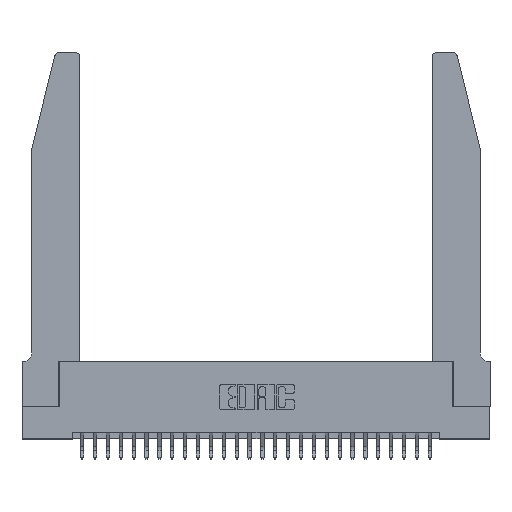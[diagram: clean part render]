
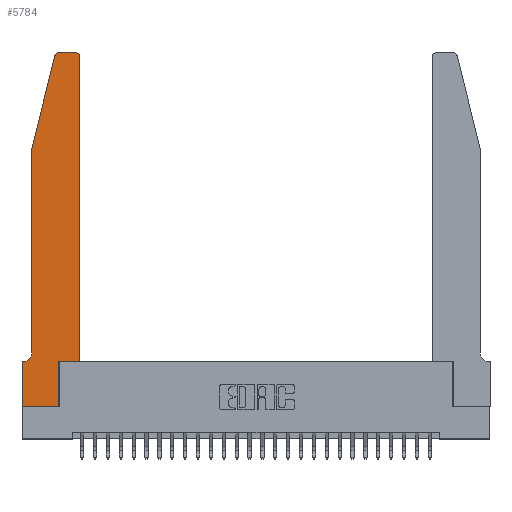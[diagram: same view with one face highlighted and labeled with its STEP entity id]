
A CAD part, top view. The second image highlights one B-rep face of the part: STEP entity #5784.
In plain terms, the highlighted planar face has unit normal (0, 0, 1).
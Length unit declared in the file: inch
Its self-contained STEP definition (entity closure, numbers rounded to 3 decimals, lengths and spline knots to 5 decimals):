
#33 = DIRECTION ( 'NONE',  ( 0., 1., 0. ) ) ;
#262 = VECTOR ( 'NONE', #13490, 39.37008 ) ;
#275 = ORIENTED_EDGE ( 'NONE', *, *, #11122, .T. ) ;
#571 = VERTEX_POINT ( 'NONE', #5229 ) ;
#741 = VERTEX_POINT ( 'NONE', #20770 ) ;
#930 = LINE ( 'NONE', #17009, #28403 ) ;
#1021 = ORIENTED_EDGE ( 'NONE', *, *, #4474, .T. ) ;
#1080 = FACE_OUTER_BOUND ( 'NONE', #5150, .T. ) ;
#1816 = CARTESIAN_POINT ( 'NONE',  ( 0.2865, 0.35, 0.37 ) ) ;
#1835 = CIRCLE ( 'NONE', #12754, 0.03 ) ;
#1891 = LINE ( 'NONE', #13065, #13332 ) ;
#2243 = LINE ( 'NONE', #26798, #19398 ) ;
#4474 = EDGE_CURVE ( 'NONE', #21054, #741, #24254, .T. ) ;
#4695 = CARTESIAN_POINT ( 'NONE',  ( 0., 0.35, 0.37 ) ) ;
#5145 = ORIENTED_EDGE ( 'NONE', *, *, #24065, .T. ) ;
#5150 = EDGE_LOOP ( 'NONE', ( #5145, #16934, #22730, #275, #1021, #7296, #18976, #20340, #15926, #21708, #11509, #28837 ) ) ;
#5229 = CARTESIAN_POINT ( 'NONE',  ( 0.4505, 0.35, 0.37 ) ) ;
#5756 = VECTOR ( 'NONE', #20949, 39.37008 ) ;
#5784 = ADVANCED_FACE ( 'NONE', ( #1080 ), #17998, .T. ) ;
#6334 = CARTESIAN_POINT ( 'NONE',  ( 0.4205, 2.72, 0.37 ) ) ;
#6457 = EDGE_CURVE ( 'NONE', #17022, #22166, #13598, .T. ) ;
#7056 = CARTESIAN_POINT ( 'NONE',  ( 0.0755, 2., 0.37 ) ) ;
#7296 = ORIENTED_EDGE ( 'NONE', *, *, #10731, .T. ) ;
#7402 = CIRCLE ( 'NONE', #26269, 0.03 ) ;
#7629 = VECTOR ( 'NONE', #26615, 39.37008 ) ;
#7757 = CARTESIAN_POINT ( 'NONE',  ( 0.4505, 0.35, 0.37 ) ) ;
#8223 = CARTESIAN_POINT ( 'NONE',  ( 0., 0.35, 0.37 ) ) ;
#8578 = DIRECTION ( 'NONE',  ( 1., 0., 0. ) ) ;
#9175 = CARTESIAN_POINT ( 'NONE',  ( 0.4505, 2.72, 0.37 ) ) ;
#9250 = DIRECTION ( 'NONE',  ( 0., 0., 1. ) ) ;
#9281 = DIRECTION ( 'NONE',  ( 0., -1., 0. ) ) ;
#9647 = EDGE_CURVE ( 'NONE', #571, #27584, #28255, .T. ) ;
#10397 = CARTESIAN_POINT ( 'NONE',  ( 0.0755, 0.42, 0.37 ) ) ;
#10710 = VERTEX_POINT ( 'NONE', #22911 ) ;
#10731 = EDGE_CURVE ( 'NONE', #741, #17732, #26187, .T. ) ;
#10800 = CARTESIAN_POINT ( 'NONE',  ( 0.0755, 2., 0.37 ) ) ;
#11122 = EDGE_CURVE ( 'NONE', #22166, #21054, #15287, .T. ) ;
#11227 = CARTESIAN_POINT ( 'NONE',  ( 0., 0., 0.37 ) ) ;
#11301 = CARTESIAN_POINT ( 'NONE',  ( 0.0755, 2., 0.37 ) ) ;
#11402 = CARTESIAN_POINT ( 'NONE',  ( 0.0055, 0.42, 0.37 ) ) ;
#11509 = ORIENTED_EDGE ( 'NONE', *, *, #9647, .T. ) ;
#11668 = EDGE_CURVE ( 'NONE', #17732, #14678, #12518, .T. ) ;
#12518 = LINE ( 'NONE', #11227, #262 ) ;
#12657 = DIRECTION ( 'NONE',  ( 1., 0., 0. ) ) ;
#12754 = AXIS2_PLACEMENT_3D ( 'NONE', #6334, #21676, #8578 ) ;
#13065 = CARTESIAN_POINT ( 'NONE',  ( 0.2605, 2.75, 0.37 ) ) ;
#13214 = CARTESIAN_POINT ( 'NONE',  ( 0.284, 2.72, 0.37 ) ) ;
#13332 = VECTOR ( 'NONE', #23901, 39.37008 ) ;
#13468 = EDGE_CURVE ( 'NONE', #22896, #571, #17512, .T. ) ;
#13490 = DIRECTION ( 'NONE',  ( 0., -1., 0. ) ) ;
#13598 = LINE ( 'NONE', #11301, #7629 ) ;
#13644 = DIRECTION ( 'NONE',  ( -1., 0., 0. ) ) ;
#13723 = AXIS2_PLACEMENT_3D ( 'NONE', #4695, #9250, #24584 ) ;
#14387 = CARTESIAN_POINT ( 'NONE',  ( 0., 0., 0.37 ) ) ;
#14611 = VECTOR ( 'NONE', #9281, 39.37008 ) ;
#14678 = VERTEX_POINT ( 'NONE', #14387 ) ;
#15287 = LINE ( 'NONE', #7056, #14611 ) ;
#15385 = DIRECTION ( 'NONE',  ( 1., 0., 0. ) ) ;
#15926 = ORIENTED_EDGE ( 'NONE', *, *, #24286, .T. ) ;
#16827 = CARTESIAN_POINT ( 'NONE',  ( 0.25487, 2.72718, 0.37 ) ) ;
#16934 = ORIENTED_EDGE ( 'NONE', *, *, #17890, .T. ) ;
#17009 = CARTESIAN_POINT ( 'NONE',  ( 0., 0., 0.37 ) ) ;
#17022 = VERTEX_POINT ( 'NONE', #16827 ) ;
#17398 = VECTOR ( 'NONE', #23135, 39.37008 ) ;
#17512 = LINE ( 'NONE', #18769, #5756 ) ;
#17590 = AXIS2_PLACEMENT_3D ( 'NONE', #11402, #26620, #13644 ) ;
#17732 = VERTEX_POINT ( 'NONE', #8223 ) ;
#17890 = EDGE_CURVE ( 'NONE', #10710, #17022, #7402, .T. ) ;
#17998 = PLANE ( 'NONE',  #13723 ) ;
#18326 = VERTEX_POINT ( 'NONE', #25449 ) ;
#18769 = CARTESIAN_POINT ( 'NONE',  ( 0.4505, 0.35, 0.37 ) ) ;
#18976 = ORIENTED_EDGE ( 'NONE', *, *, #11668, .T. ) ;
#19398 = VECTOR ( 'NONE', #33, 39.37008 ) ;
#20340 = ORIENTED_EDGE ( 'NONE', *, *, #21065, .T. ) ;
#20770 = CARTESIAN_POINT ( 'NONE',  ( 0.0055, 0.35, 0.37 ) ) ;
#20784 = DIRECTION ( 'NONE',  ( -1., 0., 0. ) ) ;
#20949 = DIRECTION ( 'NONE',  ( 1., 0., 0. ) ) ;
#21054 = VERTEX_POINT ( 'NONE', #10397 ) ;
#21065 = EDGE_CURVE ( 'NONE', #14678, #22758, #930, .T. ) ;
#21435 = CARTESIAN_POINT ( 'NONE',  ( 0.2865, 0., 0.37 ) ) ;
#21676 = DIRECTION ( 'NONE',  ( 0., 0., 1. ) ) ;
#21708 = ORIENTED_EDGE ( 'NONE', *, *, #13468, .T. ) ;
#22166 = VERTEX_POINT ( 'NONE', #10800 ) ;
#22730 = ORIENTED_EDGE ( 'NONE', *, *, #6457, .T. ) ;
#22758 = VERTEX_POINT ( 'NONE', #21435 ) ;
#22896 = VERTEX_POINT ( 'NONE', #1816 ) ;
#22911 = CARTESIAN_POINT ( 'NONE',  ( 0.284, 2.75, 0.37 ) ) ;
#23135 = DIRECTION ( 'NONE',  ( 0., 1., 0. ) ) ;
#23901 = DIRECTION ( 'NONE',  ( -1., 0., 0. ) ) ;
#24065 = EDGE_CURVE ( 'NONE', #18326, #10710, #1891, .T. ) ;
#24254 = CIRCLE ( 'NONE', #17590, 0.07 ) ;
#24286 = EDGE_CURVE ( 'NONE', #22758, #22896, #2243, .T. ) ;
#24584 = DIRECTION ( 'NONE',  ( 1., 0., 0. ) ) ;
#24829 = VECTOR ( 'NONE', #20784, 39.37008 ) ;
#25195 = CARTESIAN_POINT ( 'NONE',  ( 0.0755, 0.35, 0.37 ) ) ;
#25449 = CARTESIAN_POINT ( 'NONE',  ( 0.4205, 2.75, 0.37 ) ) ;
#25752 = EDGE_CURVE ( 'NONE', #27584, #18326, #1835, .T. ) ;
#26187 = LINE ( 'NONE', #25195, #24829 ) ;
#26269 = AXIS2_PLACEMENT_3D ( 'NONE', #13214, #28367, #15385 ) ;
#26615 = DIRECTION ( 'NONE',  ( -0.239, -0.971, 0. ) ) ;
#26620 = DIRECTION ( 'NONE',  ( 0., 0., -1. ) ) ;
#26798 = CARTESIAN_POINT ( 'NONE',  ( 0.2865, 0.35, 0.37 ) ) ;
#27584 = VERTEX_POINT ( 'NONE', #9175 ) ;
#28255 = LINE ( 'NONE', #7757, #17398 ) ;
#28367 = DIRECTION ( 'NONE',  ( 0., 0., 1. ) ) ;
#28403 = VECTOR ( 'NONE', #12657, 39.37008 ) ;
#28837 = ORIENTED_EDGE ( 'NONE', *, *, #25752, .T. ) ;
